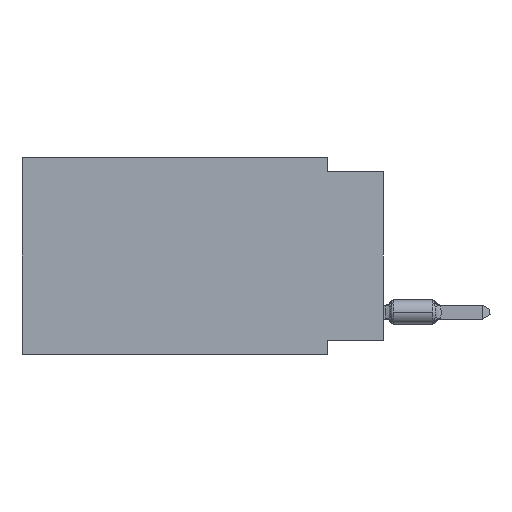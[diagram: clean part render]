
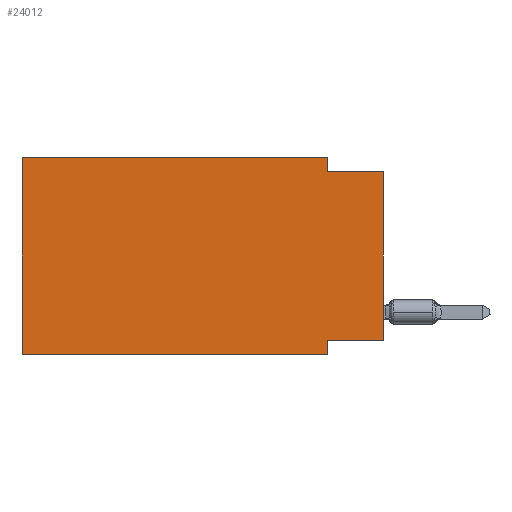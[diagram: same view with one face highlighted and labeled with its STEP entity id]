
A CAD part, left-side view. The second image highlights one B-rep face of the part: STEP entity #24012.
In plain terms, the highlighted planar face has unit normal (-1, 0, 0).
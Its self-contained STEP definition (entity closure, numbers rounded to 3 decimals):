
#843 = VECTOR ( 'NONE', #8164, 1000. ) ;
#1267 = VERTEX_POINT ( 'NONE', #31377 ) ;
#1739 = DIRECTION ( 'NONE',  ( 0., 0., -1. ) ) ;
#1966 = FACE_OUTER_BOUND ( 'NONE', #26423, .T. ) ;
#2129 = CARTESIAN_POINT ( 'NONE',  ( 0., 0., -8.255 ) ) ;
#2431 = VERTEX_POINT ( 'NONE', #11444 ) ;
#2710 = VECTOR ( 'NONE', #44190, 1000. ) ;
#2883 = DIRECTION ( 'NONE',  ( 1., 0., 0. ) ) ;
#3764 = VERTEX_POINT ( 'NONE', #39603 ) ;
#4342 = DIRECTION ( 'NONE',  ( 0., -1., 0. ) ) ;
#5795 = EDGE_CURVE ( 'NONE', #34692, #20755, #5993, .T. ) ;
#5993 = LINE ( 'NONE', #6667, #37138 ) ;
#6148 = CARTESIAN_POINT ( 'NONE',  ( 0., 16.383, 0. ) ) ;
#6312 = LINE ( 'NONE', #13399, #2710 ) ;
#6375 = DIRECTION ( 'NONE',  ( 0., 0., -1. ) ) ;
#6667 = CARTESIAN_POINT ( 'NONE',  ( 0., 2.54, -8.89 ) ) ;
#8164 = DIRECTION ( 'NONE',  ( 0., 0., 1. ) ) ;
#8675 = CARTESIAN_POINT ( 'NONE',  ( 0., 0., -0.635 ) ) ;
#9077 = VERTEX_POINT ( 'NONE', #6148 ) ;
#9523 = EDGE_CURVE ( 'NONE', #2431, #9077, #6312, .T. ) ;
#10204 = ORIENTED_EDGE ( 'NONE', *, *, #27652, .F. ) ;
#11444 = CARTESIAN_POINT ( 'NONE',  ( 0., 16.383, -8.89 ) ) ;
#12149 = VECTOR ( 'NONE', #1739, 1000. ) ;
#12491 = PLANE ( 'NONE',  #12790 ) ;
#12790 = AXIS2_PLACEMENT_3D ( 'NONE', #26393, #2883, #16138 ) ;
#13399 = CARTESIAN_POINT ( 'NONE',  ( 0., 16.383, 0. ) ) ;
#15346 = CARTESIAN_POINT ( 'NONE',  ( 0., 16.383, -8.89 ) ) ;
#15461 = CARTESIAN_POINT ( 'NONE',  ( 0., 2.54, 0. ) ) ;
#15549 = ORIENTED_EDGE ( 'NONE', *, *, #42703, .F. ) ;
#15571 = LINE ( 'NONE', #15346, #18779 ) ;
#16138 = DIRECTION ( 'NONE',  ( 0., 0., -1. ) ) ;
#16389 = ORIENTED_EDGE ( 'NONE', *, *, #41902, .F. ) ;
#16799 = EDGE_CURVE ( 'NONE', #3764, #23274, #33006, .T. ) ;
#17019 = CARTESIAN_POINT ( 'NONE',  ( 0., 2.54, 0. ) ) ;
#17632 = EDGE_CURVE ( 'NONE', #26658, #1267, #42603, .T. ) ;
#17668 = CARTESIAN_POINT ( 'NONE',  ( 0., 0., -0.635 ) ) ;
#18779 = VECTOR ( 'NONE', #29258, 1000. ) ;
#19661 = DIRECTION ( 'NONE',  ( 0., -1., 0. ) ) ;
#20755 = VERTEX_POINT ( 'NONE', #28410 ) ;
#21213 = ORIENTED_EDGE ( 'NONE', *, *, #17632, .F. ) ;
#21917 = LINE ( 'NONE', #8675, #26706 ) ;
#22866 = VECTOR ( 'NONE', #33169, 1000. ) ;
#23274 = VERTEX_POINT ( 'NONE', #17668 ) ;
#24012 = ADVANCED_FACE ( 'NONE', ( #1966 ), #12491, .F. ) ;
#26393 = CARTESIAN_POINT ( 'NONE',  ( 0., 16.383, 0. ) ) ;
#26423 = EDGE_LOOP ( 'NONE', ( #30401, #10204, #21213, #16389, #27428, #33643, #40842, #15549 ) ) ;
#26658 = VERTEX_POINT ( 'NONE', #17019 ) ;
#26706 = VECTOR ( 'NONE', #4342, 1000. ) ;
#26763 = VECTOR ( 'NONE', #19661, 1000. ) ;
#27428 = ORIENTED_EDGE ( 'NONE', *, *, #9523, .F. ) ;
#27652 = EDGE_CURVE ( 'NONE', #1267, #23274, #21917, .T. ) ;
#28410 = CARTESIAN_POINT ( 'NONE',  ( 0., 2.54, -8.89 ) ) ;
#29258 = DIRECTION ( 'NONE',  ( 0., -1., 0. ) ) ;
#30142 = LINE ( 'NONE', #44285, #26763 ) ;
#30401 = ORIENTED_EDGE ( 'NONE', *, *, #16799, .T. ) ;
#31377 = CARTESIAN_POINT ( 'NONE',  ( 0., 2.54, -0.635 ) ) ;
#33006 = LINE ( 'NONE', #43277, #843 ) ;
#33169 = DIRECTION ( 'NONE',  ( 0., 1., 0. ) ) ;
#33643 = ORIENTED_EDGE ( 'NONE', *, *, #41756, .T. ) ;
#34692 = VERTEX_POINT ( 'NONE', #42435 ) ;
#37138 = VECTOR ( 'NONE', #6375, 1000. ) ;
#39603 = CARTESIAN_POINT ( 'NONE',  ( 0., 0., -8.255 ) ) ;
#40704 = LINE ( 'NONE', #2129, #22866 ) ;
#40842 = ORIENTED_EDGE ( 'NONE', *, *, #5795, .F. ) ;
#41756 = EDGE_CURVE ( 'NONE', #2431, #20755, #15571, .T. ) ;
#41902 = EDGE_CURVE ( 'NONE', #9077, #26658, #30142, .T. ) ;
#42435 = CARTESIAN_POINT ( 'NONE',  ( 0., 2.54, -8.255 ) ) ;
#42603 = LINE ( 'NONE', #15461, #12149 ) ;
#42703 = EDGE_CURVE ( 'NONE', #3764, #34692, #40704, .T. ) ;
#43277 = CARTESIAN_POINT ( 'NONE',  ( 0., 0., 0. ) ) ;
#44190 = DIRECTION ( 'NONE',  ( 0., 0., 1. ) ) ;
#44285 = CARTESIAN_POINT ( 'NONE',  ( 0., 16.383, 0. ) ) ;
